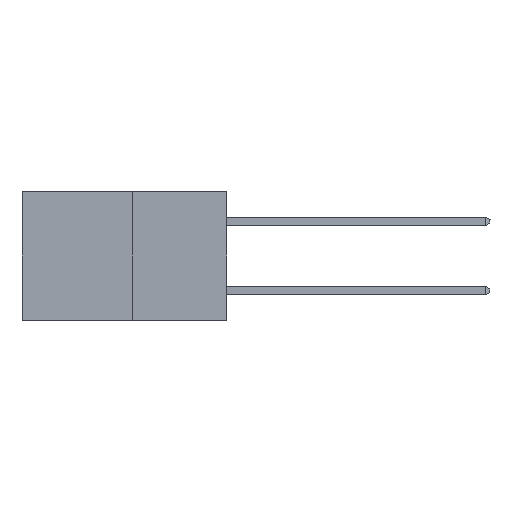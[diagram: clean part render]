
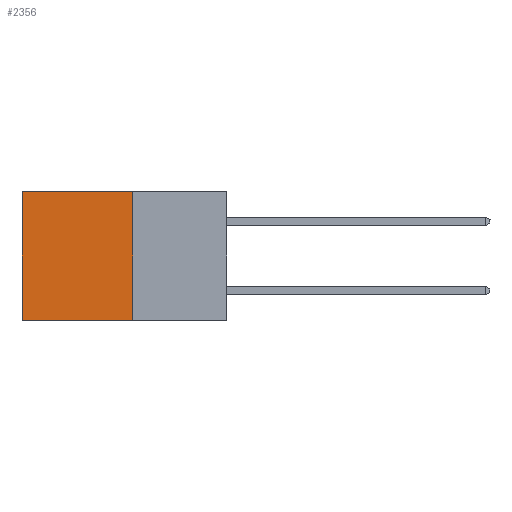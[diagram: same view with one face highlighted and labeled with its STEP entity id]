
A CAD part, left-side view. The second image highlights one B-rep face of the part: STEP entity #2356.
In plain terms, the highlighted planar face has unit normal (-1, 0, 0).
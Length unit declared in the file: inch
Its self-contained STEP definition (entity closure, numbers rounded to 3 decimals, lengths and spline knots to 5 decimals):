
#692 = VERTEX_POINT ( 'NONE', #4279 ) ;
#841 = CARTESIAN_POINT ( 'NONE',  ( 0.277, 0.59, 0. ) ) ;
#877 = VECTOR ( 'NONE', #1651, 39.37008 ) ;
#1016 = CARTESIAN_POINT ( 'NONE',  ( 0.277, 0.27, -0.37 ) ) ;
#1063 = EDGE_CURVE ( 'NONE', #7697, #7268, #5574, .T. ) ;
#1293 = CARTESIAN_POINT ( 'NONE',  ( 0.277, 0.27, 0. ) ) ;
#1369 = ORIENTED_EDGE ( 'NONE', *, *, #1063, .F. ) ;
#1440 = EDGE_CURVE ( 'NONE', #692, #4432, #1453, .T. ) ;
#1453 = LINE ( 'NONE', #1293, #8091 ) ;
#1651 = DIRECTION ( 'NONE',  ( 0., 0., -1. ) ) ;
#1666 = DIRECTION ( 'NONE',  ( 0., 1., 0. ) ) ;
#1783 = VECTOR ( 'NONE', #5082, 39.37008 ) ;
#2304 = DIRECTION ( 'NONE',  ( 0., 0., -1. ) ) ;
#2356 = ADVANCED_FACE ( 'NONE', ( #5455 ), #7277, .F. ) ;
#2873 = ORIENTED_EDGE ( 'NONE', *, *, #1440, .T. ) ;
#3801 = VECTOR ( 'NONE', #1666, 39.37008 ) ;
#4279 = CARTESIAN_POINT ( 'NONE',  ( 0.277, 0.27, 0. ) ) ;
#4432 = VERTEX_POINT ( 'NONE', #841 ) ;
#4614 = ORIENTED_EDGE ( 'NONE', *, *, #5926, .T. ) ;
#4843 = DIRECTION ( 'NONE',  ( 0., 1., 0. ) ) ;
#4879 = CARTESIAN_POINT ( 'NONE',  ( 0.277, 0.59, -0.37 ) ) ;
#5082 = DIRECTION ( 'NONE',  ( 0., 0., -1. ) ) ;
#5129 = CARTESIAN_POINT ( 'NONE',  ( 0.277, 0.59, -0.37 ) ) ;
#5455 = FACE_OUTER_BOUND ( 'NONE', #6726, .T. ) ;
#5574 = LINE ( 'NONE', #7940, #3801 ) ;
#5649 = ORIENTED_EDGE ( 'NONE', *, *, #7682, .F. ) ;
#5926 = EDGE_CURVE ( 'NONE', #4432, #7268, #7008, .T. ) ;
#6183 = LINE ( 'NONE', #1016, #877 ) ;
#6248 = AXIS2_PLACEMENT_3D ( 'NONE', #7143, #6930, #2304 ) ;
#6726 = EDGE_LOOP ( 'NONE', ( #4614, #1369, #5649, #2873 ) ) ;
#6908 = CARTESIAN_POINT ( 'NONE',  ( 0.277, 0.27, -0.37 ) ) ;
#6930 = DIRECTION ( 'NONE',  ( 1., 0., 0. ) ) ;
#7008 = LINE ( 'NONE', #5129, #1783 ) ;
#7143 = CARTESIAN_POINT ( 'NONE',  ( 0.277, 0.27, -0.37 ) ) ;
#7268 = VERTEX_POINT ( 'NONE', #4879 ) ;
#7277 = PLANE ( 'NONE',  #6248 ) ;
#7682 = EDGE_CURVE ( 'NONE', #692, #7697, #6183, .T. ) ;
#7697 = VERTEX_POINT ( 'NONE', #6908 ) ;
#7940 = CARTESIAN_POINT ( 'NONE',  ( 0.277, 0.27, -0.37 ) ) ;
#8091 = VECTOR ( 'NONE', #4843, 39.37008 ) ;
